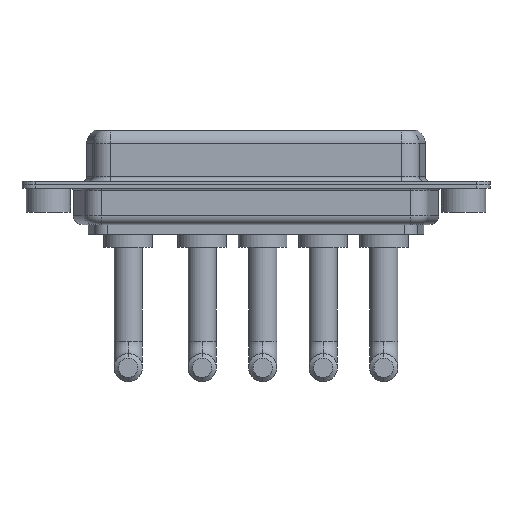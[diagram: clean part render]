
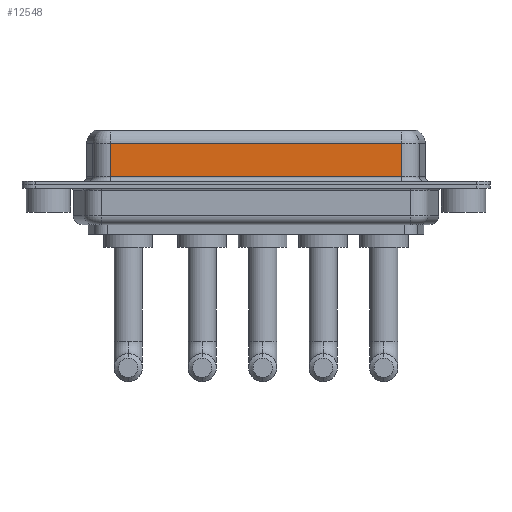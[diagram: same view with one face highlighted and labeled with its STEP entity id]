
A CAD part, front view. The second image highlights one B-rep face of the part: STEP entity #12548.
In plain terms, the highlighted planar face has unit normal (0, -1, 0).
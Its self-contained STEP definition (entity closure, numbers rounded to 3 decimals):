
#203 = DIRECTION ( 'NONE',  ( 0., 0., -1. ) ) ;
#432 = VERTEX_POINT ( 'NONE', #8270 ) ;
#509 = DIRECTION ( 'NONE',  ( -1., 0., 0. ) ) ;
#751 = CARTESIAN_POINT ( 'NONE',  ( 40.037, -3.95, 6.4 ) ) ;
#1008 = CARTESIAN_POINT ( 'NONE',  ( 40.037, -3.95, 6.4 ) ) ;
#1785 = DIRECTION ( 'NONE',  ( 0., 0., 1. ) ) ;
#2139 = CARTESIAN_POINT ( 'NONE',  ( 7.013, -3.95, 6.4 ) ) ;
#2258 = LINE ( 'NONE', #7941, #3470 ) ;
#2431 = CARTESIAN_POINT ( 'NONE',  ( 7.013, -3.95, 4.65 ) ) ;
#2469 = EDGE_LOOP ( 'NONE', ( #2640, #11489, #5452, #11269 ) ) ;
#2470 = VERTEX_POINT ( 'NONE', #2431 ) ;
#2640 = ORIENTED_EDGE ( 'NONE', *, *, #3360, .F. ) ;
#2951 = LINE ( 'NONE', #1008, #4089 ) ;
#3054 = EDGE_CURVE ( 'NONE', #432, #3404, #2258, .T. ) ;
#3360 = EDGE_CURVE ( 'NONE', #11815, #3404, #2951, .T. ) ;
#3404 = VERTEX_POINT ( 'NONE', #8697 ) ;
#3470 = VECTOR ( 'NONE', #8130, 1000. ) ;
#4089 = VECTOR ( 'NONE', #8881, 1000. ) ;
#4679 = DIRECTION ( 'NONE',  ( 0., 1., 0. ) ) ;
#5452 = ORIENTED_EDGE ( 'NONE', *, *, #9485, .T. ) ;
#6250 = VECTOR ( 'NONE', #203, 1000. ) ;
#6267 = VECTOR ( 'NONE', #509, 1000. ) ;
#6688 = PLANE ( 'NONE',  #11494 ) ;
#6751 = FACE_OUTER_BOUND ( 'NONE', #2469, .T. ) ;
#7941 = CARTESIAN_POINT ( 'NONE',  ( 40.037, -3.95, 0.9 ) ) ;
#8130 = DIRECTION ( 'NONE',  ( 1., 0., 0. ) ) ;
#8270 = CARTESIAN_POINT ( 'NONE',  ( 7.013, -3.95, 0.9 ) ) ;
#8697 = CARTESIAN_POINT ( 'NONE',  ( 40.037, -3.95, 0.9 ) ) ;
#8881 = DIRECTION ( 'NONE',  ( 0., 0., -1. ) ) ;
#9271 = CARTESIAN_POINT ( 'NONE',  ( 40.037, -3.95, 4.65 ) ) ;
#9485 = EDGE_CURVE ( 'NONE', #2470, #432, #12015, .T. ) ;
#10442 = EDGE_CURVE ( 'NONE', #11815, #2470, #10969, .T. ) ;
#10445 = CARTESIAN_POINT ( 'NONE',  ( 40.037, -3.95, 4.65 ) ) ;
#10969 = LINE ( 'NONE', #10445, #6267 ) ;
#11269 = ORIENTED_EDGE ( 'NONE', *, *, #3054, .T. ) ;
#11489 = ORIENTED_EDGE ( 'NONE', *, *, #10442, .T. ) ;
#11494 = AXIS2_PLACEMENT_3D ( 'NONE', #751, #4679, #1785 ) ;
#11815 = VERTEX_POINT ( 'NONE', #9271 ) ;
#12015 = LINE ( 'NONE', #2139, #6250 ) ;
#12548 = ADVANCED_FACE ( 'NONE', ( #6751 ), #6688, .F. ) ;
